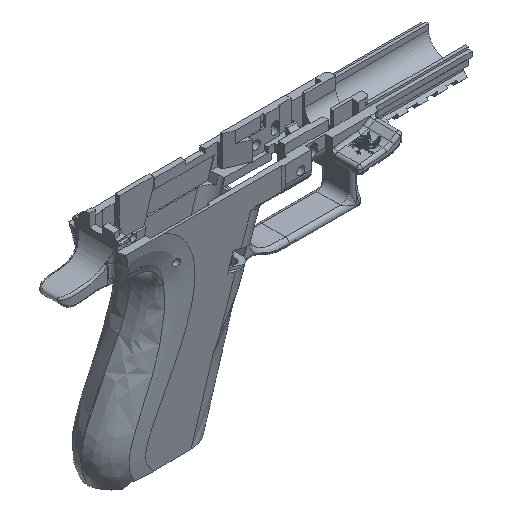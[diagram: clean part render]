
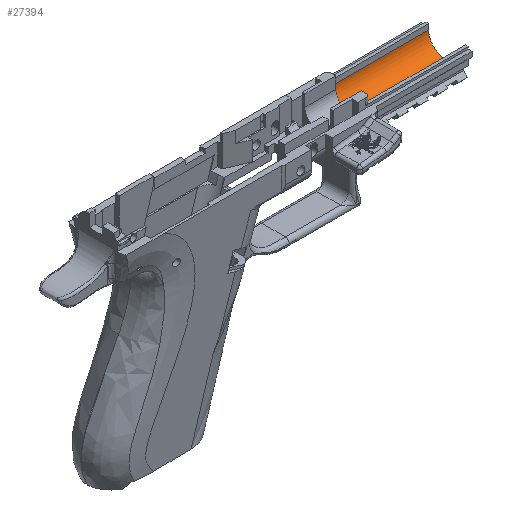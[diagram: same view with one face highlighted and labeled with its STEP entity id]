
A CAD part, isometric view. The second image highlights one B-rep face of the part: STEP entity #27394.
In plain terms, the highlighted cylindrical face has radius 8.75 mm (diameter 17.5 mm), a partial arc.
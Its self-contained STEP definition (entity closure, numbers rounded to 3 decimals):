
#132=CYLINDRICAL_SURFACE('',#28197,8.75);
#3318=LINE('',#60655,#5297);
#3320=LINE('',#60665,#5299);
#5297=VECTOR('',#31447,1000.);
#5299=VECTOR('',#31451,1000.);
#7584=FACE_OUTER_BOUND('',#9077,.T.);
#9077=EDGE_LOOP('',(#25032,#25033,#25034,#25035,#25036));
#9389=CIRCLE('',#28059,8.75);
#9418=CIRCLE('',#28198,8.75);
#10514=B_SPLINE_CURVE_WITH_KNOTS('',3,(#60658,#60659,#60660,#60661,#60662,
#60663),.UNSPECIFIED.,.F.,.F.,(4,2,4),(0.734,0.932,
1.014),.UNSPECIFIED.);
#13106=VERTEX_POINT('',#59949);
#13107=VERTEX_POINT('',#59950);
#13272=VERTEX_POINT('',#60652);
#13273=VERTEX_POINT('',#60654);
#13274=VERTEX_POINT('',#60664);
#17040=EDGE_CURVE('',#13106,#13107,#9389,.T.);
#17327=EDGE_CURVE('',#13273,#13272,#3318,.T.);
#17329=EDGE_CURVE('',#13272,#13106,#10514,.T.);
#17330=EDGE_CURVE('',#13274,#13107,#3320,.T.);
#17331=EDGE_CURVE('',#13273,#13274,#9418,.T.);
#25032=ORIENTED_EDGE('',*,*,#17327,.T.);
#25033=ORIENTED_EDGE('',*,*,#17329,.T.);
#25034=ORIENTED_EDGE('',*,*,#17040,.T.);
#25035=ORIENTED_EDGE('',*,*,#17330,.F.);
#25036=ORIENTED_EDGE('',*,*,#17331,.F.);
#27394=ADVANCED_FACE('',(#7584),#132,.F.);
#28059=AXIS2_PLACEMENT_3D('',#59951,#30935,#30936);
#28197=AXIS2_PLACEMENT_3D('',#60657,#31449,#31450);
#28198=AXIS2_PLACEMENT_3D('',#60666,#31452,#31453);
#30935=DIRECTION('center_axis',(-1.,0.,0.));
#30936=DIRECTION('ref_axis',(0.,-1.,0.));
#31447=DIRECTION('',(-1.,0.,0.));
#31449=DIRECTION('center_axis',(-1.,0.,0.));
#31450=DIRECTION('ref_axis',(0.,-1.,0.));
#31451=DIRECTION('',(-1.,0.,0.));
#31452=DIRECTION('center_axis',(-1.,0.,0.));
#31453=DIRECTION('ref_axis',(0.,-1.,0.));
#59949=CARTESIAN_POINT('',(128.4,33.743,102.843));
#59950=CARTESIAN_POINT('',(128.4,25.493,97.009));
#59951=CARTESIAN_POINT('Origin',(128.4,25.493,105.759));
#60652=CARTESIAN_POINT('',(128.336,34.243,105.759));
#60654=CARTESIAN_POINT('',(178.4,34.243,105.759));
#60655=CARTESIAN_POINT('',(178.4,34.243,105.759));
#60657=CARTESIAN_POINT('Origin',(178.4,25.493,105.759));
#60658=CARTESIAN_POINT('Ctrl Pts',(128.336,34.243,105.759));
#60659=CARTESIAN_POINT('Ctrl Pts',(128.336,34.243,105.099));
#60660=CARTESIAN_POINT('Ctrl Pts',(128.363,34.163,104.382));
#60661=CARTESIAN_POINT('Ctrl Pts',(128.393,33.924,103.402));
#60662=CARTESIAN_POINT('Ctrl Pts',(128.4,33.84,103.118));
#60663=CARTESIAN_POINT('Ctrl Pts',(128.4,33.743,102.843));
#60664=CARTESIAN_POINT('',(178.4,25.493,97.009));
#60665=CARTESIAN_POINT('',(178.4,25.493,97.009));
#60666=CARTESIAN_POINT('Origin',(178.4,25.493,105.759));
